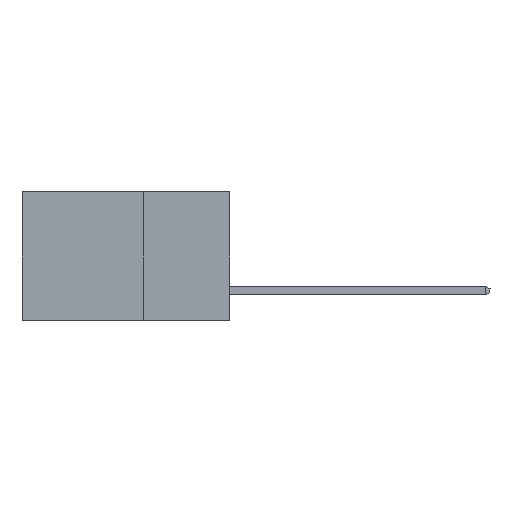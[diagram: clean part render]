
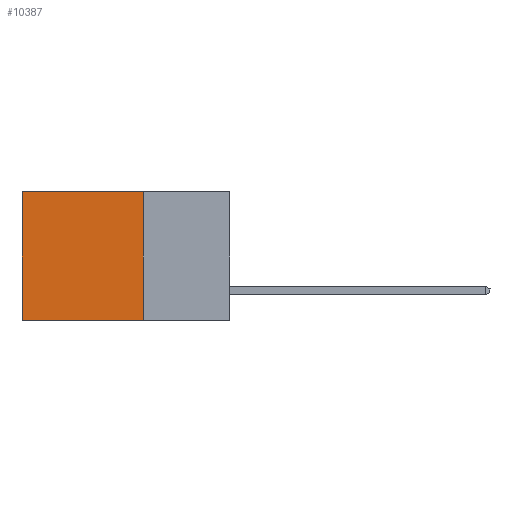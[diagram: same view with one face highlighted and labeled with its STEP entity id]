
A CAD part, left-side view. The second image highlights one B-rep face of the part: STEP entity #10387.
In plain terms, the highlighted planar face has unit normal (-1, 0, 0).
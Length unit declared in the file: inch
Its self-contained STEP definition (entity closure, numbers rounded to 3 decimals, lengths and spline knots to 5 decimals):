
#135 = PLANE ( 'NONE',  #3198 ) ;
#659 = LINE ( 'NONE', #6343, #7309 ) ;
#847 = EDGE_CURVE ( 'NONE', #4500, #11067, #6863, .T. ) ;
#969 = ORIENTED_EDGE ( 'NONE', *, *, #5139, .F. ) ;
#1116 = ORIENTED_EDGE ( 'NONE', *, *, #847, .F. ) ;
#1501 = EDGE_CURVE ( 'NONE', #6597, #3940, #659, .T. ) ;
#1785 = DIRECTION ( 'NONE',  ( 0., 0., -1. ) ) ;
#1794 = CARTESIAN_POINT ( 'NONE',  ( 0.2615, 0.25, -0.37 ) ) ;
#2117 = LINE ( 'NONE', #11648, #7600 ) ;
#2403 = VECTOR ( 'NONE', #2465, 39.37008 ) ;
#2465 = DIRECTION ( 'NONE',  ( 0., 1., 0. ) ) ;
#3144 = DIRECTION ( 'NONE',  ( 0., 1., 0. ) ) ;
#3198 = AXIS2_PLACEMENT_3D ( 'NONE', #9811, #6008, #5879 ) ;
#3940 = VERTEX_POINT ( 'NONE', #7851 ) ;
#4139 = EDGE_LOOP ( 'NONE', ( #4315, #969, #1116, #5613 ) ) ;
#4195 = LINE ( 'NONE', #11851, #2403 ) ;
#4315 = ORIENTED_EDGE ( 'NONE', *, *, #1501, .T. ) ;
#4500 = VERTEX_POINT ( 'NONE', #10478 ) ;
#5139 = EDGE_CURVE ( 'NONE', #11067, #3940, #2117, .T. ) ;
#5613 = ORIENTED_EDGE ( 'NONE', *, *, #7098, .T. ) ;
#5790 = DIRECTION ( 'NONE',  ( 0., 0., -1. ) ) ;
#5879 = DIRECTION ( 'NONE',  ( 0., 0., -1. ) ) ;
#6008 = DIRECTION ( 'NONE',  ( 1., 0., 0. ) ) ;
#6343 = CARTESIAN_POINT ( 'NONE',  ( 0.2615, 0.6, -0.37 ) ) ;
#6597 = VERTEX_POINT ( 'NONE', #9980 ) ;
#6821 = FACE_OUTER_BOUND ( 'NONE', #4139, .T. ) ;
#6863 = LINE ( 'NONE', #6921, #9501 ) ;
#6921 = CARTESIAN_POINT ( 'NONE',  ( 0.2615, 0.25, -0.37 ) ) ;
#7098 = EDGE_CURVE ( 'NONE', #4500, #6597, #4195, .T. ) ;
#7309 = VECTOR ( 'NONE', #1785, 39.37008 ) ;
#7600 = VECTOR ( 'NONE', #3144, 39.37008 ) ;
#7851 = CARTESIAN_POINT ( 'NONE',  ( 0.2615, 0.6, -0.37 ) ) ;
#9501 = VECTOR ( 'NONE', #5790, 39.37008 ) ;
#9811 = CARTESIAN_POINT ( 'NONE',  ( 0.2615, 0.25, -0.37 ) ) ;
#9980 = CARTESIAN_POINT ( 'NONE',  ( 0.2615, 0.6, 0. ) ) ;
#10387 = ADVANCED_FACE ( 'NONE', ( #6821 ), #135, .F. ) ;
#10478 = CARTESIAN_POINT ( 'NONE',  ( 0.2615, 0.25, 0. ) ) ;
#11067 = VERTEX_POINT ( 'NONE', #1794 ) ;
#11648 = CARTESIAN_POINT ( 'NONE',  ( 0.2615, 0.25, -0.37 ) ) ;
#11851 = CARTESIAN_POINT ( 'NONE',  ( 0.2615, 0.25, 0. ) ) ;
